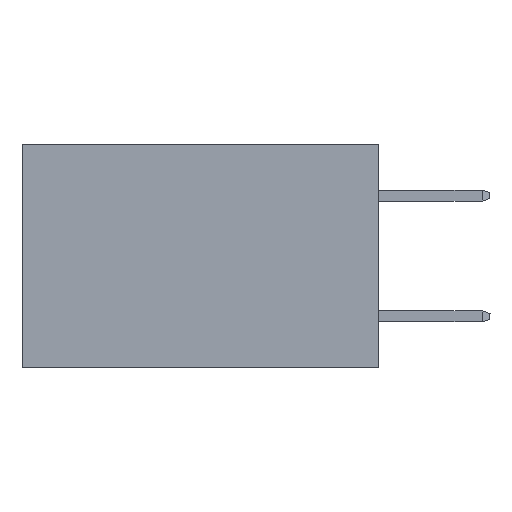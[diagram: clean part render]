
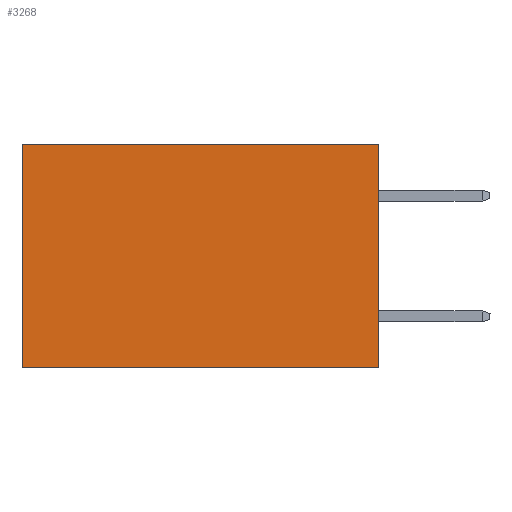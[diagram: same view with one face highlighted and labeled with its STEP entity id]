
A CAD part, left-side view. The second image highlights one B-rep face of the part: STEP entity #3268.
In plain terms, the highlighted planar face has unit normal (-1, 0, 0).
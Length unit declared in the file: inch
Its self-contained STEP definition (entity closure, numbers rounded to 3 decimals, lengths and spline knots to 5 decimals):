
#254 = VECTOR ( 'NONE', #309, 39.37008 ) ;
#309 = DIRECTION ( 'NONE',  ( 0., 0., -1. ) ) ;
#623 = LINE ( 'NONE', #8002, #254 ) ;
#666 = ORIENTED_EDGE ( 'NONE', *, *, #5273, .F. ) ;
#912 = CARTESIAN_POINT ( 'NONE',  ( 0.277, 0., -0.37 ) ) ;
#1112 = DIRECTION ( 'NONE',  ( 0., 0., -1. ) ) ;
#1127 = CARTESIAN_POINT ( 'NONE',  ( 0.277, 0., -0.37 ) ) ;
#1492 = CARTESIAN_POINT ( 'NONE',  ( 0.277, 0., -0.37 ) ) ;
#1710 = CARTESIAN_POINT ( 'NONE',  ( 0.277, 0., 0. ) ) ;
#1813 = CARTESIAN_POINT ( 'NONE',  ( 0.277, 0.59, -0.37 ) ) ;
#2183 = LINE ( 'NONE', #6489, #5597 ) ;
#3087 = FACE_OUTER_BOUND ( 'NONE', #3569, .T. ) ;
#3214 = AXIS2_PLACEMENT_3D ( 'NONE', #912, #5516, #7141 ) ;
#3268 = ADVANCED_FACE ( 'NONE', ( #3087 ), #3661, .F. ) ;
#3569 = EDGE_LOOP ( 'NONE', ( #7392, #666, #4458, #6124 ) ) ;
#3661 = PLANE ( 'NONE',  #3214 ) ;
#4085 = VECTOR ( 'NONE', #7336, 39.37008 ) ;
#4458 = ORIENTED_EDGE ( 'NONE', *, *, #6608, .F. ) ;
#5055 = VERTEX_POINT ( 'NONE', #1710 ) ;
#5273 = EDGE_CURVE ( 'NONE', #6408, #8080, #5783, .T. ) ;
#5516 = DIRECTION ( 'NONE',  ( 1., 0., 0. ) ) ;
#5571 = VERTEX_POINT ( 'NONE', #5582 ) ;
#5577 = VECTOR ( 'NONE', #1112, 39.37008 ) ;
#5582 = CARTESIAN_POINT ( 'NONE',  ( 0.277, 0.59, 0. ) ) ;
#5597 = VECTOR ( 'NONE', #7064, 39.37008 ) ;
#5756 = LINE ( 'NONE', #1127, #5577 ) ;
#5783 = LINE ( 'NONE', #7408, #4085 ) ;
#6124 = ORIENTED_EDGE ( 'NONE', *, *, #8097, .T. ) ;
#6408 = VERTEX_POINT ( 'NONE', #1492 ) ;
#6489 = CARTESIAN_POINT ( 'NONE',  ( 0.277, 0., 0. ) ) ;
#6608 = EDGE_CURVE ( 'NONE', #5055, #6408, #5756, .T. ) ;
#7064 = DIRECTION ( 'NONE',  ( 0., 1., 0. ) ) ;
#7141 = DIRECTION ( 'NONE',  ( 0., 0., -1. ) ) ;
#7336 = DIRECTION ( 'NONE',  ( 0., 1., 0. ) ) ;
#7392 = ORIENTED_EDGE ( 'NONE', *, *, #7973, .T. ) ;
#7408 = CARTESIAN_POINT ( 'NONE',  ( 0.277, 0., -0.37 ) ) ;
#7973 = EDGE_CURVE ( 'NONE', #5571, #8080, #623, .T. ) ;
#8002 = CARTESIAN_POINT ( 'NONE',  ( 0.277, 0.59, -0.37 ) ) ;
#8080 = VERTEX_POINT ( 'NONE', #1813 ) ;
#8097 = EDGE_CURVE ( 'NONE', #5055, #5571, #2183, .T. ) ;
